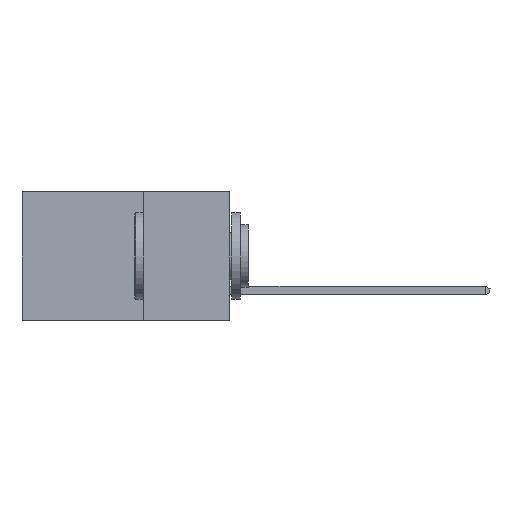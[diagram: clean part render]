
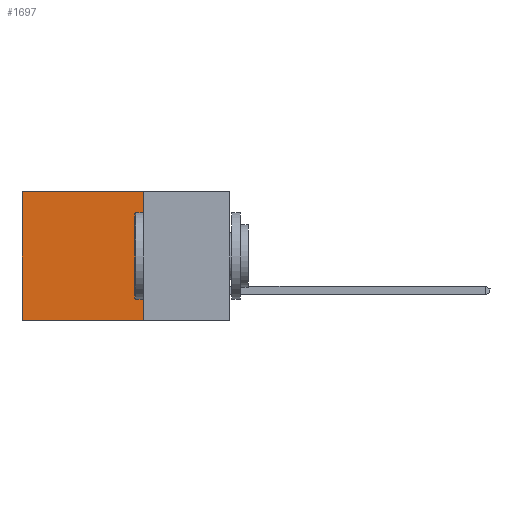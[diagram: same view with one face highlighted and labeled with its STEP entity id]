
A CAD part, left-side view. The second image highlights one B-rep face of the part: STEP entity #1697.
In plain terms, the highlighted planar face has unit normal (-1, 0, 0).
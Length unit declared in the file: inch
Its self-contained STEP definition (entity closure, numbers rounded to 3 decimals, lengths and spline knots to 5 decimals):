
#390 = LINE ( 'NONE', #20572, #11849 ) ;
#1314 = CARTESIAN_POINT ( 'NONE',  ( 0.2615, 0.6, 0. ) ) ;
#1416 = CARTESIAN_POINT ( 'NONE',  ( 0.2615, 0.25, 0. ) ) ;
#1697 = ADVANCED_FACE ( 'NONE', ( #10113 ), #10223, .F. ) ;
#1837 = CARTESIAN_POINT ( 'NONE',  ( 0.2615, 0.6, -0.37 ) ) ;
#2819 = EDGE_LOOP ( 'NONE', ( #4430, #8508, #3638, #16124 ) ) ;
#2830 = EDGE_CURVE ( 'NONE', #10735, #3735, #11240, .T. ) ;
#3638 = ORIENTED_EDGE ( 'NONE', *, *, #2830, .F. ) ;
#3735 = VERTEX_POINT ( 'NONE', #5668 ) ;
#4368 = EDGE_CURVE ( 'NONE', #10735, #15583, #22725, .T. ) ;
#4430 = ORIENTED_EDGE ( 'NONE', *, *, #21382, .T. ) ;
#5668 = CARTESIAN_POINT ( 'NONE',  ( 0.2615, 0.25, -0.37 ) ) ;
#8508 = ORIENTED_EDGE ( 'NONE', *, *, #8571, .F. ) ;
#8571 = EDGE_CURVE ( 'NONE', #3735, #17561, #390, .T. ) ;
#10113 = FACE_OUTER_BOUND ( 'NONE', #2819, .T. ) ;
#10223 = PLANE ( 'NONE',  #17315 ) ;
#10343 = DIRECTION ( 'NONE',  ( 1., 0., 0. ) ) ;
#10735 = VERTEX_POINT ( 'NONE', #16899 ) ;
#11160 = DIRECTION ( 'NONE',  ( 0., 1., 0. ) ) ;
#11240 = LINE ( 'NONE', #22228, #15422 ) ;
#11790 = CARTESIAN_POINT ( 'NONE',  ( 0.2615, 0.25, -0.37 ) ) ;
#11849 = VECTOR ( 'NONE', #11160, 39.37008 ) ;
#15422 = VECTOR ( 'NONE', #16322, 39.37008 ) ;
#15583 = VERTEX_POINT ( 'NONE', #1314 ) ;
#16124 = ORIENTED_EDGE ( 'NONE', *, *, #4368, .T. ) ;
#16322 = DIRECTION ( 'NONE',  ( 0., 0., -1. ) ) ;
#16899 = CARTESIAN_POINT ( 'NONE',  ( 0.2615, 0.25, 0. ) ) ;
#17315 = AXIS2_PLACEMENT_3D ( 'NONE', #11790, #10343, #19170 ) ;
#17561 = VERTEX_POINT ( 'NONE', #1837 ) ;
#17708 = CARTESIAN_POINT ( 'NONE',  ( 0.2615, 0.6, -0.37 ) ) ;
#17842 = DIRECTION ( 'NONE',  ( 0., 1., 0. ) ) ;
#19170 = DIRECTION ( 'NONE',  ( 0., 0., -1. ) ) ;
#20105 = VECTOR ( 'NONE', #17842, 39.37008 ) ;
#20572 = CARTESIAN_POINT ( 'NONE',  ( 0.2615, 0.25, -0.37 ) ) ;
#21092 = VECTOR ( 'NONE', #23387, 39.37008 ) ;
#21382 = EDGE_CURVE ( 'NONE', #15583, #17561, #21581, .T. ) ;
#21581 = LINE ( 'NONE', #17708, #21092 ) ;
#22228 = CARTESIAN_POINT ( 'NONE',  ( 0.2615, 0.25, -0.37 ) ) ;
#22725 = LINE ( 'NONE', #1416, #20105 ) ;
#23387 = DIRECTION ( 'NONE',  ( 0., 0., -1. ) ) ;
